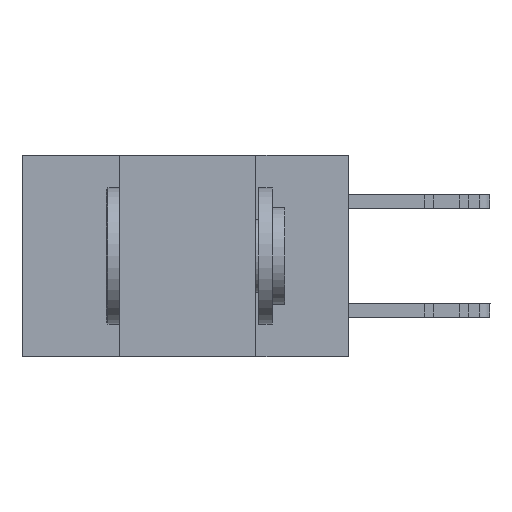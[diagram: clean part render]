
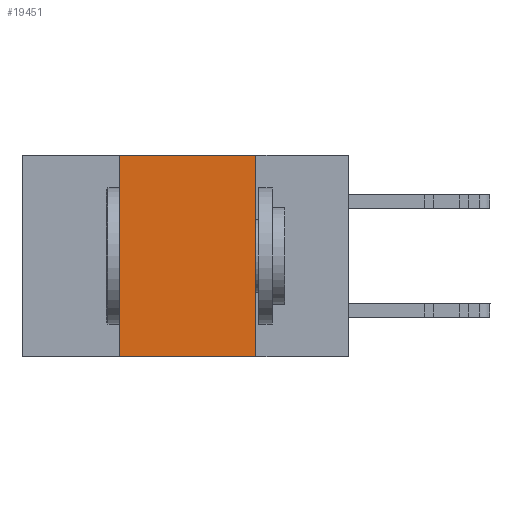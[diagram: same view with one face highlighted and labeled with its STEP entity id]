
A CAD part, left-side view. The second image highlights one B-rep face of the part: STEP entity #19451.
In plain terms, the highlighted planar face has unit normal (-1, 0, 0).
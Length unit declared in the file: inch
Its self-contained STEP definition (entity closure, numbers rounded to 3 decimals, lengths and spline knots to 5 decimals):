
#1589 = VECTOR ( 'NONE', #9434, 39.37008 ) ;
#1777 = ORIENTED_EDGE ( 'NONE', *, *, #17430, .F. ) ;
#2636 = DIRECTION ( 'NONE',  ( 0., -1., 0. ) ) ;
#2723 = VECTOR ( 'NONE', #14533, 39.37008 ) ;
#4004 = VERTEX_POINT ( 'NONE', #12515 ) ;
#4535 = DIRECTION ( 'NONE',  ( 1., 0., 0. ) ) ;
#5335 = CARTESIAN_POINT ( 'NONE',  ( 0., 0.42, -0.37 ) ) ;
#6102 = LINE ( 'NONE', #14789, #16266 ) ;
#7130 = CARTESIAN_POINT ( 'NONE',  ( 0., 0.6, 0. ) ) ;
#7489 = LINE ( 'NONE', #7130, #2723 ) ;
#7550 = EDGE_CURVE ( 'NONE', #4004, #15191, #7489, .T. ) ;
#7679 = LINE ( 'NONE', #11498, #1589 ) ;
#8024 = CARTESIAN_POINT ( 'NONE',  ( 0., 0.42, -0.37 ) ) ;
#8479 = ORIENTED_EDGE ( 'NONE', *, *, #18611, .F. ) ;
#9291 = AXIS2_PLACEMENT_3D ( 'NONE', #10528, #4535, #18754 ) ;
#9434 = DIRECTION ( 'NONE',  ( 0., 0., -1. ) ) ;
#10383 = CARTESIAN_POINT ( 'NONE',  ( 0., 0.17, -0.37 ) ) ;
#10528 = CARTESIAN_POINT ( 'NONE',  ( 0., 0.6, 0. ) ) ;
#10529 = EDGE_CURVE ( 'NONE', #23928, #23043, #6102, .T. ) ;
#11498 = CARTESIAN_POINT ( 'NONE',  ( 0., 0.17, -0.37 ) ) ;
#12246 = EDGE_LOOP ( 'NONE', ( #1777, #13265, #8479, #14215 ) ) ;
#12515 = CARTESIAN_POINT ( 'NONE',  ( 0., 0.42, 0. ) ) ;
#13265 = ORIENTED_EDGE ( 'NONE', *, *, #7550, .F. ) ;
#14215 = ORIENTED_EDGE ( 'NONE', *, *, #10529, .T. ) ;
#14277 = FACE_OUTER_BOUND ( 'NONE', #12246, .T. ) ;
#14533 = DIRECTION ( 'NONE',  ( 0., -1., 0. ) ) ;
#14639 = PLANE ( 'NONE',  #9291 ) ;
#14789 = CARTESIAN_POINT ( 'NONE',  ( 0., 0.6, -0.37 ) ) ;
#15191 = VERTEX_POINT ( 'NONE', #20954 ) ;
#16266 = VECTOR ( 'NONE', #2636, 39.37008 ) ;
#16818 = VECTOR ( 'NONE', #18264, 39.37008 ) ;
#17430 = EDGE_CURVE ( 'NONE', #15191, #23043, #7679, .T. ) ;
#18264 = DIRECTION ( 'NONE',  ( 0., 0., 1. ) ) ;
#18611 = EDGE_CURVE ( 'NONE', #23928, #4004, #22189, .T. ) ;
#18754 = DIRECTION ( 'NONE',  ( 0., 0., -1. ) ) ;
#19451 = ADVANCED_FACE ( 'NONE', ( #14277 ), #14639, .F. ) ;
#20954 = CARTESIAN_POINT ( 'NONE',  ( 0., 0.17, 0. ) ) ;
#22189 = LINE ( 'NONE', #8024, #16818 ) ;
#23043 = VERTEX_POINT ( 'NONE', #10383 ) ;
#23928 = VERTEX_POINT ( 'NONE', #5335 ) ;
